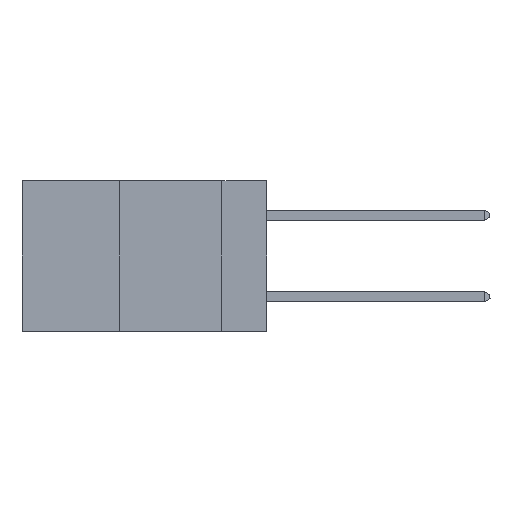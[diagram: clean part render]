
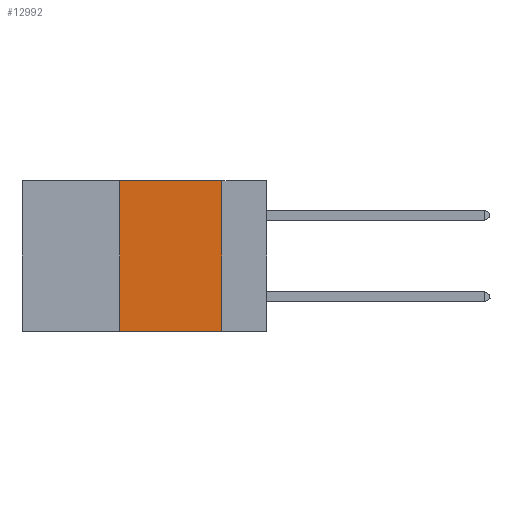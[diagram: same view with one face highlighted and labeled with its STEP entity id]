
A CAD part, left-side view. The second image highlights one B-rep face of the part: STEP entity #12992.
In plain terms, the highlighted planar face has unit normal (-1, 0, 0).
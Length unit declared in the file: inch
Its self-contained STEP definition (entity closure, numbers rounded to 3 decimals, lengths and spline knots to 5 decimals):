
#1839 = CARTESIAN_POINT ( 'NONE',  ( 0., 0.6, -0.37 ) ) ;
#3516 = VERTEX_POINT ( 'NONE', #23514 ) ;
#3810 = EDGE_CURVE ( 'NONE', #25862, #3516, #21165, .T. ) ;
#4179 = DIRECTION ( 'NONE',  ( 0., -1., 0. ) ) ;
#4567 = EDGE_CURVE ( 'NONE', #3516, #14559, #19033, .T. ) ;
#4958 = ORIENTED_EDGE ( 'NONE', *, *, #9238, .F. ) ;
#6629 = AXIS2_PLACEMENT_3D ( 'NONE', #14666, #16813, #21749 ) ;
#7097 = VECTOR ( 'NONE', #4179, 39.37008 ) ;
#7837 = DIRECTION ( 'NONE',  ( 0., 0., -1. ) ) ;
#8328 = DIRECTION ( 'NONE',  ( 0., 0., 1. ) ) ;
#9070 = LINE ( 'NONE', #14167, #26344 ) ;
#9238 = EDGE_CURVE ( 'NONE', #14559, #22436, #9070, .T. ) ;
#12814 = CARTESIAN_POINT ( 'NONE',  ( 0., 0.36, -0.37 ) ) ;
#12992 = ADVANCED_FACE ( 'NONE', ( #20509 ), #28125, .F. ) ;
#13050 = VECTOR ( 'NONE', #15564, 39.37008 ) ;
#13194 = CARTESIAN_POINT ( 'NONE',  ( 0., 0.6, 0. ) ) ;
#14167 = CARTESIAN_POINT ( 'NONE',  ( 0., 0.11, 0. ) ) ;
#14559 = VERTEX_POINT ( 'NONE', #18562 ) ;
#14666 = CARTESIAN_POINT ( 'NONE',  ( 0., 0.6, 0. ) ) ;
#15564 = DIRECTION ( 'NONE',  ( 0., -1., 0. ) ) ;
#15833 = ORIENTED_EDGE ( 'NONE', *, *, #3810, .F. ) ;
#16813 = DIRECTION ( 'NONE',  ( 1., 0., 0. ) ) ;
#17303 = CARTESIAN_POINT ( 'NONE',  ( 0., 0.36, 0. ) ) ;
#18562 = CARTESIAN_POINT ( 'NONE',  ( 0., 0.11, 0. ) ) ;
#19033 = LINE ( 'NONE', #13194, #13050 ) ;
#19149 = LINE ( 'NONE', #1839, #7097 ) ;
#20509 = FACE_OUTER_BOUND ( 'NONE', #25270, .T. ) ;
#21165 = LINE ( 'NONE', #17303, #27467 ) ;
#21749 = DIRECTION ( 'NONE',  ( 0., 0., -1. ) ) ;
#22162 = ORIENTED_EDGE ( 'NONE', *, *, #4567, .F. ) ;
#22436 = VERTEX_POINT ( 'NONE', #24466 ) ;
#22477 = EDGE_CURVE ( 'NONE', #25862, #22436, #19149, .T. ) ;
#23514 = CARTESIAN_POINT ( 'NONE',  ( 0., 0.36, 0. ) ) ;
#24466 = CARTESIAN_POINT ( 'NONE',  ( 0., 0.11, -0.37 ) ) ;
#25270 = EDGE_LOOP ( 'NONE', ( #4958, #22162, #15833, #29055 ) ) ;
#25862 = VERTEX_POINT ( 'NONE', #12814 ) ;
#26344 = VECTOR ( 'NONE', #7837, 39.37008 ) ;
#27467 = VECTOR ( 'NONE', #8328, 39.37008 ) ;
#28125 = PLANE ( 'NONE',  #6629 ) ;
#29055 = ORIENTED_EDGE ( 'NONE', *, *, #22477, .T. ) ;
